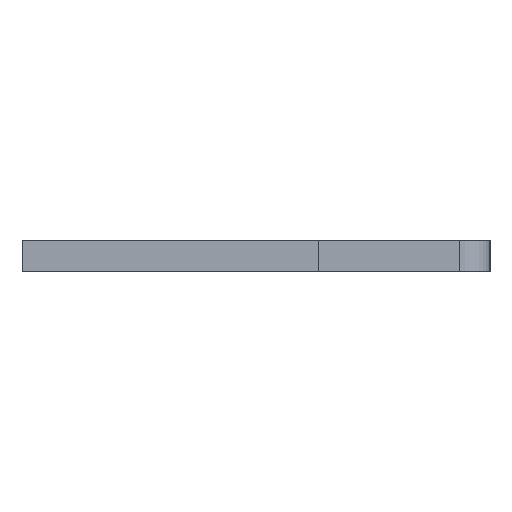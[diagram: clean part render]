
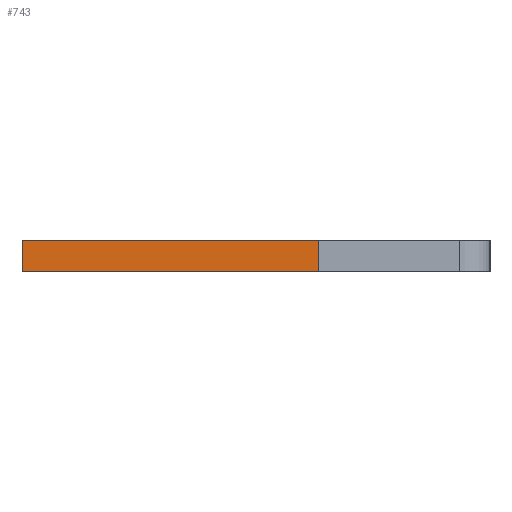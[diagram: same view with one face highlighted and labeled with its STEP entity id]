
A CAD part, left-side view. The second image highlights one B-rep face of the part: STEP entity #743.
In plain terms, the highlighted face is planar.
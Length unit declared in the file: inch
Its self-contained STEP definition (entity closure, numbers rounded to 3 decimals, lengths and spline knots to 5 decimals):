
#62 = ORIENTED_EDGE ( 'NONE', *, *, #273, .F. ) ;
#77 = DIRECTION ( 'NONE',  ( 0., 1., 0. ) ) ;
#100 = VECTOR ( 'NONE', #285, 39.37008 ) ;
#113 = PLANE ( 'NONE',  #487 ) ;
#131 = VECTOR ( 'NONE', #77, 39.37008 ) ;
#165 = EDGE_CURVE ( 'NONE', #1302, #859, #1162, .T. ) ;
#184 = CARTESIAN_POINT ( 'NONE',  ( 0.01, 0.15, -0.04 ) ) ;
#221 = DIRECTION ( 'NONE',  ( 1., 0., 0. ) ) ;
#229 = VERTEX_POINT ( 'NONE', #925 ) ;
#247 = VECTOR ( 'NONE', #717, 39.37008 ) ;
#271 = CARTESIAN_POINT ( 'NONE',  ( -0.01, 0.15, -0.04 ) ) ;
#273 = EDGE_CURVE ( 'NONE', #859, #229, #408, .T. ) ;
#285 = DIRECTION ( 'NONE',  ( -1., 0., 0. ) ) ;
#290 = EDGE_CURVE ( 'NONE', #1302, #1262, #917, .T. ) ;
#397 = CARTESIAN_POINT ( 'NONE',  ( 0.01, 0.15, -0.04 ) ) ;
#408 = LINE ( 'NONE', #397, #753 ) ;
#422 = LINE ( 'NONE', #271, #131 ) ;
#435 = EDGE_CURVE ( 'NONE', #1262, #229, #422, .T. ) ;
#463 = CARTESIAN_POINT ( 'NONE',  ( 0.01, 0.15, -0.04 ) ) ;
#487 = AXIS2_PLACEMENT_3D ( 'NONE', #463, #755, #221 ) ;
#580 = FACE_OUTER_BOUND ( 'NONE', #1076, .T. ) ;
#609 = DIRECTION ( 'NONE',  ( -1., 0., 0. ) ) ;
#717 = DIRECTION ( 'NONE',  ( 0., 1., 0. ) ) ;
#743 = ADVANCED_FACE ( 'NONE', ( #580 ), #113, .F. ) ;
#753 = VECTOR ( 'NONE', #609, 39.37008 ) ;
#755 = DIRECTION ( 'NONE',  ( 0., 0., 1. ) ) ;
#833 = CARTESIAN_POINT ( 'NONE',  ( 0.01, -0.04, -0.04 ) ) ;
#859 = VERTEX_POINT ( 'NONE', #184 ) ;
#883 = ORIENTED_EDGE ( 'NONE', *, *, #435, .T. ) ;
#917 = LINE ( 'NONE', #833, #100 ) ;
#925 = CARTESIAN_POINT ( 'NONE',  ( -0.01, 0.15, -0.04 ) ) ;
#1007 = CARTESIAN_POINT ( 'NONE',  ( 0.01, 0.15, -0.04 ) ) ;
#1076 = EDGE_LOOP ( 'NONE', ( #883, #62, #1249, #1332 ) ) ;
#1127 = CARTESIAN_POINT ( 'NONE',  ( 0.01, -0.04, -0.04 ) ) ;
#1144 = CARTESIAN_POINT ( 'NONE',  ( -0.01, -0.04, -0.04 ) ) ;
#1162 = LINE ( 'NONE', #1007, #247 ) ;
#1249 = ORIENTED_EDGE ( 'NONE', *, *, #165, .F. ) ;
#1262 = VERTEX_POINT ( 'NONE', #1144 ) ;
#1302 = VERTEX_POINT ( 'NONE', #1127 ) ;
#1332 = ORIENTED_EDGE ( 'NONE', *, *, #290, .T. ) ;
